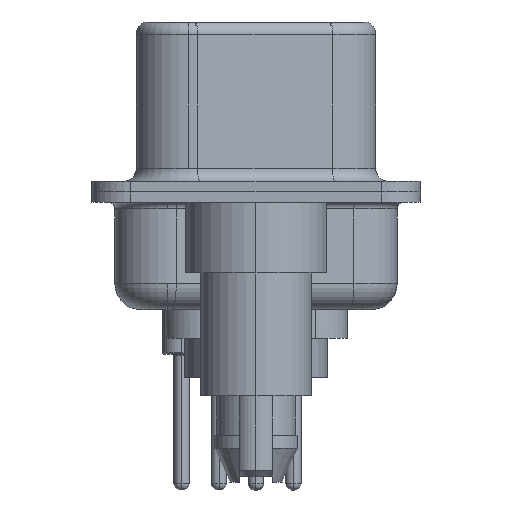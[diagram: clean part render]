
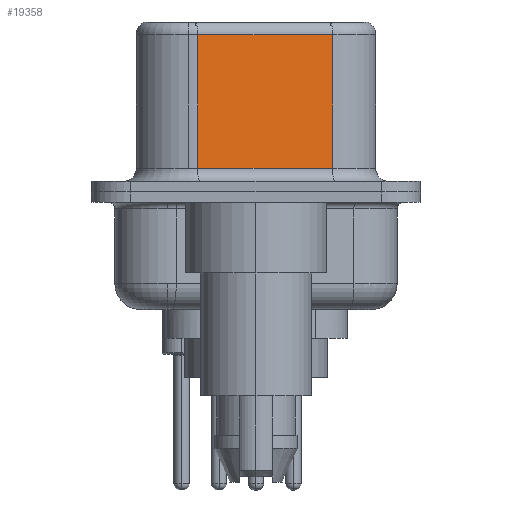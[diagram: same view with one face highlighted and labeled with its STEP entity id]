
A CAD part, left-side view. The second image highlights one B-rep face of the part: STEP entity #19358.
In plain terms, the highlighted planar face has unit normal (-0.985, -0.174, 0).
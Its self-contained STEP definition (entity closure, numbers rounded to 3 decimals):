
#159 = VECTOR ( 'NONE', #17183, 1000. ) ;
#914 = DIRECTION ( 'NONE',  ( -0.174, 0.985, 0. ) ) ;
#1132 = AXIS2_PLACEMENT_3D ( 'NONE', #27711, #17037, #4256 ) ;
#1136 = CARTESIAN_POINT ( 'NONE',  ( 4.58, -2.927, 6.02 ) ) ;
#1928 = PLANE ( 'NONE',  #1132 ) ;
#1993 = EDGE_CURVE ( 'NONE', #23229, #18471, #11885, .T. ) ;
#2632 = DIRECTION ( 'NONE',  ( 0.174, -0.985, 0. ) ) ;
#3504 = EDGE_CURVE ( 'NONE', #19011, #11386, #17196, .T. ) ;
#4256 = DIRECTION ( 'NONE',  ( -0.174, 0.985, 0. ) ) ;
#5900 = DIRECTION ( 'NONE',  ( 0., 0., -1. ) ) ;
#6397 = ORIENTED_EDGE ( 'NONE', *, *, #12509, .T. ) ;
#7374 = CARTESIAN_POINT ( 'NONE',  ( 4.58, -2.927, 6.52 ) ) ;
#10232 = ORIENTED_EDGE ( 'NONE', *, *, #20643, .T. ) ;
#11386 = VERTEX_POINT ( 'NONE', #21834 ) ;
#11885 = LINE ( 'NONE', #7374, #27646 ) ;
#12509 = EDGE_CURVE ( 'NONE', #11386, #18471, #16056, .T. ) ;
#13680 = CARTESIAN_POINT ( 'NONE',  ( 4.58, -2.927, 6.02 ) ) ;
#14323 = ORIENTED_EDGE ( 'NONE', *, *, #1993, .F. ) ;
#15792 = CARTESIAN_POINT ( 'NONE',  ( 3.67, 2.233, 6.02 ) ) ;
#16056 = LINE ( 'NONE', #21914, #26824 ) ;
#17037 = DIRECTION ( 'NONE',  ( 0.985, 0.174, 0. ) ) ;
#17183 = DIRECTION ( 'NONE',  ( 0., 0., -1. ) ) ;
#17196 = LINE ( 'NONE', #17332, #159 ) ;
#17332 = CARTESIAN_POINT ( 'NONE',  ( 3.67, 2.233, 6.52 ) ) ;
#18471 = VERTEX_POINT ( 'NONE', #27054 ) ;
#19011 = VERTEX_POINT ( 'NONE', #15792 ) ;
#19358 = ADVANCED_FACE ( 'NONE', ( #23877 ), #1928, .F. ) ;
#20643 = EDGE_CURVE ( 'NONE', #23229, #19011, #22539, .T. ) ;
#21834 = CARTESIAN_POINT ( 'NONE',  ( 3.67, 2.233, 0.9 ) ) ;
#21914 = CARTESIAN_POINT ( 'NONE',  ( 4.58, -2.927, 0.9 ) ) ;
#22182 = ORIENTED_EDGE ( 'NONE', *, *, #3504, .T. ) ;
#22539 = LINE ( 'NONE', #13680, #23201 ) ;
#23201 = VECTOR ( 'NONE', #914, 1000. ) ;
#23229 = VERTEX_POINT ( 'NONE', #1136 ) ;
#23877 = FACE_OUTER_BOUND ( 'NONE', #24649, .T. ) ;
#24649 = EDGE_LOOP ( 'NONE', ( #14323, #10232, #22182, #6397 ) ) ;
#26824 = VECTOR ( 'NONE', #2632, 1000. ) ;
#27054 = CARTESIAN_POINT ( 'NONE',  ( 4.58, -2.927, 0.9 ) ) ;
#27646 = VECTOR ( 'NONE', #5900, 1000. ) ;
#27711 = CARTESIAN_POINT ( 'NONE',  ( 4.58, -2.927, 6.52 ) ) ;
